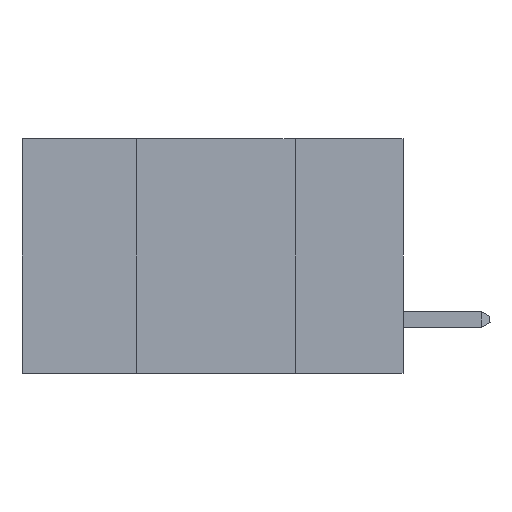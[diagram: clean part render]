
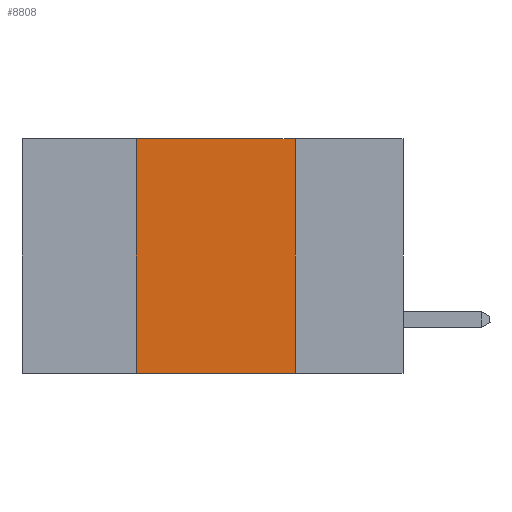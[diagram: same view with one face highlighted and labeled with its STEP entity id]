
A CAD part, left-side view. The second image highlights one B-rep face of the part: STEP entity #8808.
In plain terms, the highlighted planar face has unit normal (-1, 0, 0).
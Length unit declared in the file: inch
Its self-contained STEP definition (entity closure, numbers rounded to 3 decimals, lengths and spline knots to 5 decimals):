
#1649 = CARTESIAN_POINT ( 'NONE',  ( 0., 0.42, 0. ) ) ;
#3337 = CARTESIAN_POINT ( 'NONE',  ( 0., 0.17, -0.37 ) ) ;
#3879 = DIRECTION ( 'NONE',  ( 0., 0., 1. ) ) ;
#3989 = DIRECTION ( 'NONE',  ( 1., 0., 0. ) ) ;
#5772 = FACE_OUTER_BOUND ( 'NONE', #13737, .T. ) ;
#5917 = CARTESIAN_POINT ( 'NONE',  ( 0., 0.42, 0. ) ) ;
#6248 = VERTEX_POINT ( 'NONE', #5917 ) ;
#6310 = EDGE_CURVE ( 'NONE', #19865, #6248, #17597, .T. ) ;
#8808 = ADVANCED_FACE ( 'NONE', ( #5772 ), #15151, .F. ) ;
#10034 = DIRECTION ( 'NONE',  ( 0., 0., -1. ) ) ;
#10479 = AXIS2_PLACEMENT_3D ( 'NONE', #12151, #3989, #10034 ) ;
#10516 = LINE ( 'NONE', #27182, #27499 ) ;
#11484 = CARTESIAN_POINT ( 'NONE',  ( 0., 0.6, 0. ) ) ;
#12151 = CARTESIAN_POINT ( 'NONE',  ( 0., 0.6, 0. ) ) ;
#13737 = EDGE_LOOP ( 'NONE', ( #15638, #20481, #25160, #21534 ) ) ;
#14091 = DIRECTION ( 'NONE',  ( 0., -1., 0. ) ) ;
#15139 = VECTOR ( 'NONE', #18395, 39.37008 ) ;
#15151 = PLANE ( 'NONE',  #10479 ) ;
#15638 = ORIENTED_EDGE ( 'NONE', *, *, #26383, .F. ) ;
#15967 = CARTESIAN_POINT ( 'NONE',  ( 0., 0.42, -0.37 ) ) ;
#16209 = VECTOR ( 'NONE', #3879, 39.37008 ) ;
#17597 = LINE ( 'NONE', #1649, #16209 ) ;
#18395 = DIRECTION ( 'NONE',  ( 0., 0., -1. ) ) ;
#19411 = VERTEX_POINT ( 'NONE', #28249 ) ;
#19865 = VERTEX_POINT ( 'NONE', #15967 ) ;
#20291 = LINE ( 'NONE', #11484, #26218 ) ;
#20464 = EDGE_CURVE ( 'NONE', #19865, #23637, #10516, .T. ) ;
#20481 = ORIENTED_EDGE ( 'NONE', *, *, #26893, .F. ) ;
#21534 = ORIENTED_EDGE ( 'NONE', *, *, #20464, .T. ) ;
#21699 = LINE ( 'NONE', #25077, #15139 ) ;
#23637 = VERTEX_POINT ( 'NONE', #3337 ) ;
#25077 = CARTESIAN_POINT ( 'NONE',  ( 0., 0.17, 0. ) ) ;
#25160 = ORIENTED_EDGE ( 'NONE', *, *, #6310, .F. ) ;
#26218 = VECTOR ( 'NONE', #26979, 39.37008 ) ;
#26383 = EDGE_CURVE ( 'NONE', #19411, #23637, #21699, .T. ) ;
#26893 = EDGE_CURVE ( 'NONE', #6248, #19411, #20291, .T. ) ;
#26979 = DIRECTION ( 'NONE',  ( 0., -1., 0. ) ) ;
#27182 = CARTESIAN_POINT ( 'NONE',  ( 0., 0.6, -0.37 ) ) ;
#27499 = VECTOR ( 'NONE', #14091, 39.37008 ) ;
#28249 = CARTESIAN_POINT ( 'NONE',  ( 0., 0.17, 0. ) ) ;
